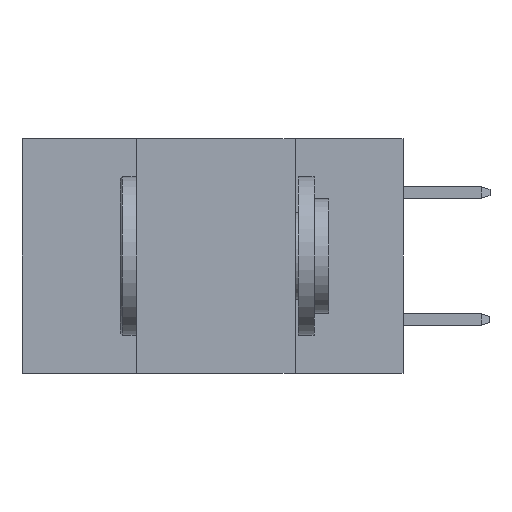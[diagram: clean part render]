
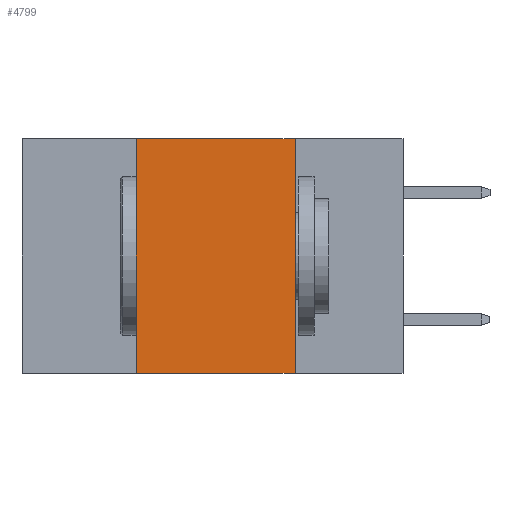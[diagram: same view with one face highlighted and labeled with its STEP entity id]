
A CAD part, left-side view. The second image highlights one B-rep face of the part: STEP entity #4799.
In plain terms, the highlighted planar face has unit normal (-1, 0, 0).
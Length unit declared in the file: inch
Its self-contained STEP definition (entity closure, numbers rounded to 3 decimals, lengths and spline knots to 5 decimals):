
#835 = CARTESIAN_POINT ( 'NONE',  ( 0., 0.42, 0. ) ) ;
#1767 = PLANE ( 'NONE',  #5039 ) ;
#1857 = CARTESIAN_POINT ( 'NONE',  ( 0., 0.17, 0. ) ) ;
#2616 = DIRECTION ( 'NONE',  ( 1., 0., 0. ) ) ;
#2733 = VECTOR ( 'NONE', #8998, 39.37008 ) ;
#3130 = EDGE_CURVE ( 'NONE', #5650, #8735, #11934, .T. ) ;
#3432 = DIRECTION ( 'NONE',  ( 0., 0., -1. ) ) ;
#4191 = EDGE_CURVE ( 'NONE', #8735, #11448, #8369, .T. ) ;
#4407 = CARTESIAN_POINT ( 'NONE',  ( 0., 0.42, -0.37 ) ) ;
#4417 = VECTOR ( 'NONE', #3432, 39.37008 ) ;
#4678 = VERTEX_POINT ( 'NONE', #4407 ) ;
#4799 = ADVANCED_FACE ( 'NONE', ( #5784 ), #1767, .F. ) ;
#5039 = AXIS2_PLACEMENT_3D ( 'NONE', #9736, #2616, #10730 ) ;
#5299 = ORIENTED_EDGE ( 'NONE', *, *, #9668, .F. ) ;
#5650 = VERTEX_POINT ( 'NONE', #835 ) ;
#5784 = FACE_OUTER_BOUND ( 'NONE', #12937, .T. ) ;
#6075 = EDGE_CURVE ( 'NONE', #4678, #11448, #10804, .T. ) ;
#6563 = ORIENTED_EDGE ( 'NONE', *, *, #6075, .T. ) ;
#7014 = CARTESIAN_POINT ( 'NONE',  ( 0., 0.17, -0.37 ) ) ;
#7887 = CARTESIAN_POINT ( 'NONE',  ( 0., 0.6, -0.37 ) ) ;
#8369 = LINE ( 'NONE', #8425, #4417 ) ;
#8425 = CARTESIAN_POINT ( 'NONE',  ( 0., 0.17, 0. ) ) ;
#8735 = VERTEX_POINT ( 'NONE', #1857 ) ;
#8944 = CARTESIAN_POINT ( 'NONE',  ( 0., 0.42, 0. ) ) ;
#8998 = DIRECTION ( 'NONE',  ( 0., 0., 1. ) ) ;
#9668 = EDGE_CURVE ( 'NONE', #4678, #5650, #11005, .T. ) ;
#9705 = VECTOR ( 'NONE', #9868, 39.37008 ) ;
#9736 = CARTESIAN_POINT ( 'NONE',  ( 0., 0.6, 0. ) ) ;
#9868 = DIRECTION ( 'NONE',  ( 0., -1., 0. ) ) ;
#10431 = ORIENTED_EDGE ( 'NONE', *, *, #3130, .F. ) ;
#10730 = DIRECTION ( 'NONE',  ( 0., 0., -1. ) ) ;
#10804 = LINE ( 'NONE', #7887, #9705 ) ;
#10928 = DIRECTION ( 'NONE',  ( 0., -1., 0. ) ) ;
#10996 = CARTESIAN_POINT ( 'NONE',  ( 0., 0.6, 0. ) ) ;
#11005 = LINE ( 'NONE', #8944, #2733 ) ;
#11345 = ORIENTED_EDGE ( 'NONE', *, *, #4191, .F. ) ;
#11448 = VERTEX_POINT ( 'NONE', #7014 ) ;
#11934 = LINE ( 'NONE', #10996, #12622 ) ;
#12622 = VECTOR ( 'NONE', #10928, 39.37008 ) ;
#12937 = EDGE_LOOP ( 'NONE', ( #11345, #10431, #5299, #6563 ) ) ;
